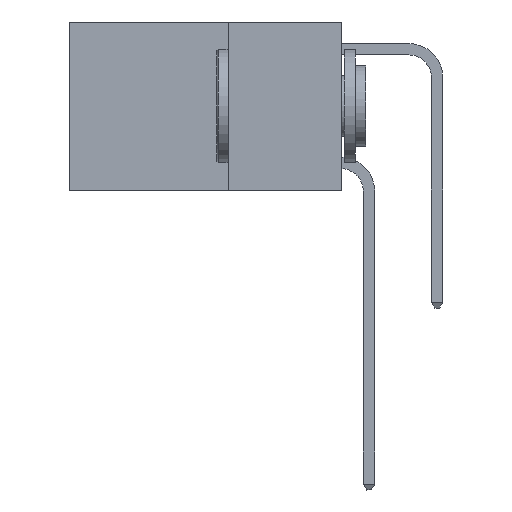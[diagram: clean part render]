
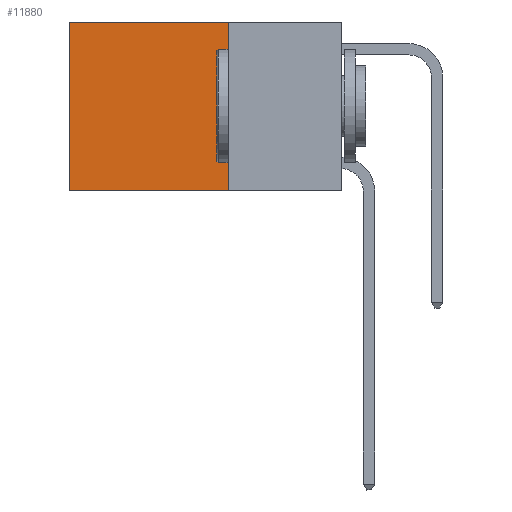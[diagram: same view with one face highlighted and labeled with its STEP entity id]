
A CAD part, left-side view. The second image highlights one B-rep face of the part: STEP entity #11880.
In plain terms, the highlighted planar face has unit normal (-1, 0, 0).
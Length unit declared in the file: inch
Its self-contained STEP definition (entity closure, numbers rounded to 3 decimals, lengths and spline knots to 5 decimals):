
#362 = AXIS2_PLACEMENT_3D ( 'NONE', #20488, #5206, #10018 ) ;
#465 = CARTESIAN_POINT ( 'NONE',  ( 0.2625, 0.25, -0.37 ) ) ;
#983 = VECTOR ( 'NONE', #11303, 39.37008 ) ;
#1433 = LINE ( 'NONE', #1989, #4299 ) ;
#1989 = CARTESIAN_POINT ( 'NONE',  ( 0.2625, 0.6, 0. ) ) ;
#2424 = CARTESIAN_POINT ( 'NONE',  ( 0.2625, 0.6, 0. ) ) ;
#2852 = VECTOR ( 'NONE', #10943, 39.37008 ) ;
#2989 = ORIENTED_EDGE ( 'NONE', *, *, #4346, .T. ) ;
#3060 = CARTESIAN_POINT ( 'NONE',  ( 0.2625, 0.25, 0. ) ) ;
#4299 = VECTOR ( 'NONE', #13685, 39.37008 ) ;
#4346 = EDGE_CURVE ( 'NONE', #18586, #14023, #14978, .T. ) ;
#5206 = DIRECTION ( 'NONE',  ( 1., 0., 0. ) ) ;
#5512 = CARTESIAN_POINT ( 'NONE',  ( 0.2625, 0.6, -0.37 ) ) ;
#5578 = LINE ( 'NONE', #465, #2852 ) ;
#6248 = DIRECTION ( 'NONE',  ( 0., 0., -1. ) ) ;
#7593 = ORIENTED_EDGE ( 'NONE', *, *, #8531, .F. ) ;
#8437 = VERTEX_POINT ( 'NONE', #15607 ) ;
#8531 = EDGE_CURVE ( 'NONE', #18586, #8437, #9374, .T. ) ;
#9374 = LINE ( 'NONE', #14499, #16672 ) ;
#9686 = EDGE_CURVE ( 'NONE', #8437, #14440, #5578, .T. ) ;
#10018 = DIRECTION ( 'NONE',  ( 0., 0., -1. ) ) ;
#10535 = EDGE_CURVE ( 'NONE', #14023, #14440, #1433, .T. ) ;
#10943 = DIRECTION ( 'NONE',  ( 0., 1., 0. ) ) ;
#11303 = DIRECTION ( 'NONE',  ( 0., 1., 0. ) ) ;
#11880 = ADVANCED_FACE ( 'NONE', ( #13364 ), #20152, .F. ) ;
#13364 = FACE_OUTER_BOUND ( 'NONE', #14756, .T. ) ;
#13685 = DIRECTION ( 'NONE',  ( 0., 0., -1. ) ) ;
#14023 = VERTEX_POINT ( 'NONE', #2424 ) ;
#14440 = VERTEX_POINT ( 'NONE', #5512 ) ;
#14499 = CARTESIAN_POINT ( 'NONE',  ( 0.2625, 0.25, 0. ) ) ;
#14756 = EDGE_LOOP ( 'NONE', ( #17912, #17683, #7593, #2989 ) ) ;
#14978 = LINE ( 'NONE', #3060, #983 ) ;
#15607 = CARTESIAN_POINT ( 'NONE',  ( 0.2625, 0.25, -0.37 ) ) ;
#16672 = VECTOR ( 'NONE', #6248, 39.37008 ) ;
#17532 = CARTESIAN_POINT ( 'NONE',  ( 0.2625, 0.25, 0. ) ) ;
#17683 = ORIENTED_EDGE ( 'NONE', *, *, #9686, .F. ) ;
#17912 = ORIENTED_EDGE ( 'NONE', *, *, #10535, .T. ) ;
#18586 = VERTEX_POINT ( 'NONE', #17532 ) ;
#20152 = PLANE ( 'NONE',  #362 ) ;
#20488 = CARTESIAN_POINT ( 'NONE',  ( 0.2625, 0.25, 0. ) ) ;
